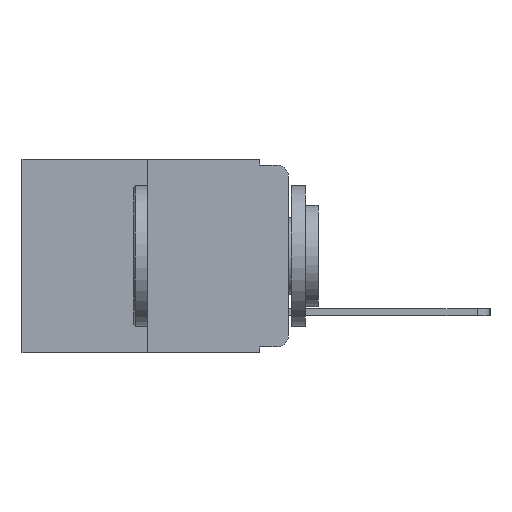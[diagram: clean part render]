
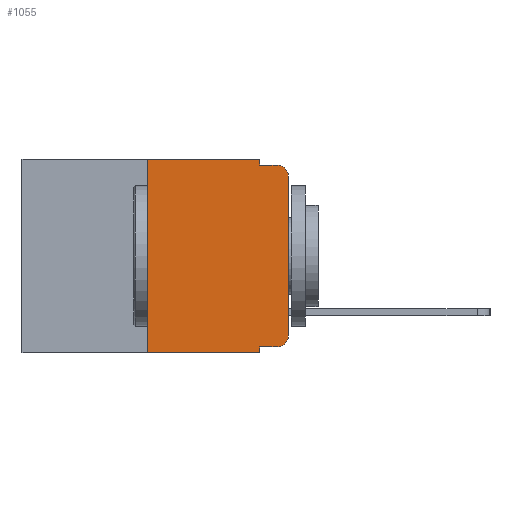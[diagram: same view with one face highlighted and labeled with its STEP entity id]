
A CAD part, left-side view. The second image highlights one B-rep face of the part: STEP entity #1055.
In plain terms, the highlighted planar face has unit normal (-1, 0, 0).
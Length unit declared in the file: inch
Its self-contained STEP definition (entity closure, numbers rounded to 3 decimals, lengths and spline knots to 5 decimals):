
#123 = LINE ( 'NONE', #11150, #10195 ) ;
#218 = LINE ( 'NONE', #2578, #11997 ) ;
#232 = EDGE_CURVE ( 'NONE', #3425, #4902, #886, .T. ) ;
#398 = CARTESIAN_POINT ( 'NONE',  ( 0., 0.051, -0.333 ) ) ;
#640 = DIRECTION ( 'NONE',  ( 0., 0., -1. ) ) ;
#723 = CARTESIAN_POINT ( 'NONE',  ( 0., 0., 0. ) ) ;
#752 = VERTEX_POINT ( 'NONE', #4450 ) ;
#770 = ORIENTED_EDGE ( 'NONE', *, *, #10401, .T. ) ;
#886 = CIRCLE ( 'NONE', #3376, 0.02 ) ;
#1055 = ADVANCED_FACE ( 'NONE', ( #3769 ), #6773, .F. ) ;
#1084 = CARTESIAN_POINT ( 'NONE',  ( 0., 0.25, -0.343 ) ) ;
#1112 = ORIENTED_EDGE ( 'NONE', *, *, #2344, .T. ) ;
#1121 = ORIENTED_EDGE ( 'NONE', *, *, #232, .T. ) ;
#1387 = DIRECTION ( 'NONE',  ( 0., 0., -1. ) ) ;
#1441 = CARTESIAN_POINT ( 'NONE',  ( 0., 0., -0.313 ) ) ;
#1456 = DIRECTION ( 'NONE',  ( 0., -1., 0. ) ) ;
#1985 = ORIENTED_EDGE ( 'NONE', *, *, #3159, .F. ) ;
#2121 = VECTOR ( 'NONE', #8502, 39.37008 ) ;
#2142 = CARTESIAN_POINT ( 'NONE',  ( 0., 0.02, -0.333 ) ) ;
#2194 = CARTESIAN_POINT ( 'NONE',  ( 0., 0., -0.03 ) ) ;
#2344 = EDGE_CURVE ( 'NONE', #5656, #3425, #4686, .T. ) ;
#2578 = CARTESIAN_POINT ( 'NONE',  ( 0., 0.25, 0. ) ) ;
#2619 = AXIS2_PLACEMENT_3D ( 'NONE', #3411, #6906, #640 ) ;
#2686 = CARTESIAN_POINT ( 'NONE',  ( 0., 0.051, 0. ) ) ;
#3122 = EDGE_CURVE ( 'NONE', #7243, #12037, #7671, .T. ) ;
#3159 = EDGE_CURVE ( 'NONE', #10165, #5583, #4823, .T. ) ;
#3363 = CIRCLE ( 'NONE', #5428, 0.02 ) ;
#3376 = AXIS2_PLACEMENT_3D ( 'NONE', #4088, #9089, #1387 ) ;
#3402 = ORIENTED_EDGE ( 'NONE', *, *, #4378, .F. ) ;
#3411 = CARTESIAN_POINT ( 'NONE',  ( 0., 0.473, 0. ) ) ;
#3425 = VERTEX_POINT ( 'NONE', #2142 ) ;
#3618 = CARTESIAN_POINT ( 'NONE',  ( 0., 0.473, -0.343 ) ) ;
#3684 = EDGE_LOOP ( 'NONE', ( #770, #5397, #10028, #12298, #1985, #3402, #3727, #9111, #1112, #1121 ) ) ;
#3697 = EDGE_CURVE ( 'NONE', #5656, #12037, #7053, .T. ) ;
#3727 = ORIENTED_EDGE ( 'NONE', *, *, #3122, .T. ) ;
#3769 = FACE_OUTER_BOUND ( 'NONE', #3684, .T. ) ;
#4008 = CARTESIAN_POINT ( 'NONE',  ( 0., 0.051, -0.01 ) ) ;
#4088 = CARTESIAN_POINT ( 'NONE',  ( 0., 0.02, -0.313 ) ) ;
#4165 = VECTOR ( 'NONE', #6639, 39.37008 ) ;
#4378 = EDGE_CURVE ( 'NONE', #7243, #10165, #218, .T. ) ;
#4427 = CARTESIAN_POINT ( 'NONE',  ( 0., 0.051, 0. ) ) ;
#4445 = CARTESIAN_POINT ( 'NONE',  ( 0., 0.25, 0. ) ) ;
#4450 = CARTESIAN_POINT ( 'NONE',  ( 0., 0.02, -0.01 ) ) ;
#4686 = LINE ( 'NONE', #398, #11694 ) ;
#4823 = LINE ( 'NONE', #5626, #2121 ) ;
#4900 = VECTOR ( 'NONE', #5285, 39.37008 ) ;
#4902 = VERTEX_POINT ( 'NONE', #1441 ) ;
#5134 = VECTOR ( 'NONE', #11945, 39.37008 ) ;
#5265 = CARTESIAN_POINT ( 'NONE',  ( 0., 0.02, -0.03 ) ) ;
#5285 = DIRECTION ( 'NONE',  ( 0., -1., 0. ) ) ;
#5397 = ORIENTED_EDGE ( 'NONE', *, *, #5469, .T. ) ;
#5428 = AXIS2_PLACEMENT_3D ( 'NONE', #5265, #11623, #6206 ) ;
#5469 = EDGE_CURVE ( 'NONE', #6156, #752, #3363, .T. ) ;
#5508 = VECTOR ( 'NONE', #10394, 39.37008 ) ;
#5583 = VERTEX_POINT ( 'NONE', #4427 ) ;
#5626 = CARTESIAN_POINT ( 'NONE',  ( 0., 0.473, 0. ) ) ;
#5656 = VERTEX_POINT ( 'NONE', #6454 ) ;
#5685 = DIRECTION ( 'NONE',  ( 0., 0., -1. ) ) ;
#5805 = LINE ( 'NONE', #723, #5508 ) ;
#6156 = VERTEX_POINT ( 'NONE', #2194 ) ;
#6206 = DIRECTION ( 'NONE',  ( 0., 0., -1. ) ) ;
#6454 = CARTESIAN_POINT ( 'NONE',  ( 0., 0.051, -0.333 ) ) ;
#6639 = DIRECTION ( 'NONE',  ( 0., 0., -1. ) ) ;
#6773 = PLANE ( 'NONE',  #2619 ) ;
#6906 = DIRECTION ( 'NONE',  ( 1., 0., 0. ) ) ;
#6968 = EDGE_CURVE ( 'NONE', #5583, #9883, #123, .T. ) ;
#7053 = LINE ( 'NONE', #2686, #4165 ) ;
#7146 = LINE ( 'NONE', #11638, #4900 ) ;
#7243 = VERTEX_POINT ( 'NONE', #1084 ) ;
#7671 = LINE ( 'NONE', #3618, #5134 ) ;
#8502 = DIRECTION ( 'NONE',  ( 0., -1., 0. ) ) ;
#9089 = DIRECTION ( 'NONE',  ( -1., 0., 0. ) ) ;
#9111 = ORIENTED_EDGE ( 'NONE', *, *, #3697, .F. ) ;
#9150 = CARTESIAN_POINT ( 'NONE',  ( 0., 0.051, -0.343 ) ) ;
#9883 = VERTEX_POINT ( 'NONE', #4008 ) ;
#10028 = ORIENTED_EDGE ( 'NONE', *, *, #10043, .F. ) ;
#10043 = EDGE_CURVE ( 'NONE', #9883, #752, #7146, .T. ) ;
#10165 = VERTEX_POINT ( 'NONE', #4445 ) ;
#10195 = VECTOR ( 'NONE', #5685, 39.37008 ) ;
#10201 = DIRECTION ( 'NONE',  ( 0., 0., 1. ) ) ;
#10394 = DIRECTION ( 'NONE',  ( 0., 0., 1. ) ) ;
#10401 = EDGE_CURVE ( 'NONE', #4902, #6156, #5805, .T. ) ;
#11150 = CARTESIAN_POINT ( 'NONE',  ( 0., 0.051, 0. ) ) ;
#11623 = DIRECTION ( 'NONE',  ( -1., 0., 0. ) ) ;
#11638 = CARTESIAN_POINT ( 'NONE',  ( 0., 0.051, -0.01 ) ) ;
#11694 = VECTOR ( 'NONE', #1456, 39.37008 ) ;
#11945 = DIRECTION ( 'NONE',  ( 0., -1., 0. ) ) ;
#11997 = VECTOR ( 'NONE', #10201, 39.37008 ) ;
#12037 = VERTEX_POINT ( 'NONE', #9150 ) ;
#12298 = ORIENTED_EDGE ( 'NONE', *, *, #6968, .F. ) ;
